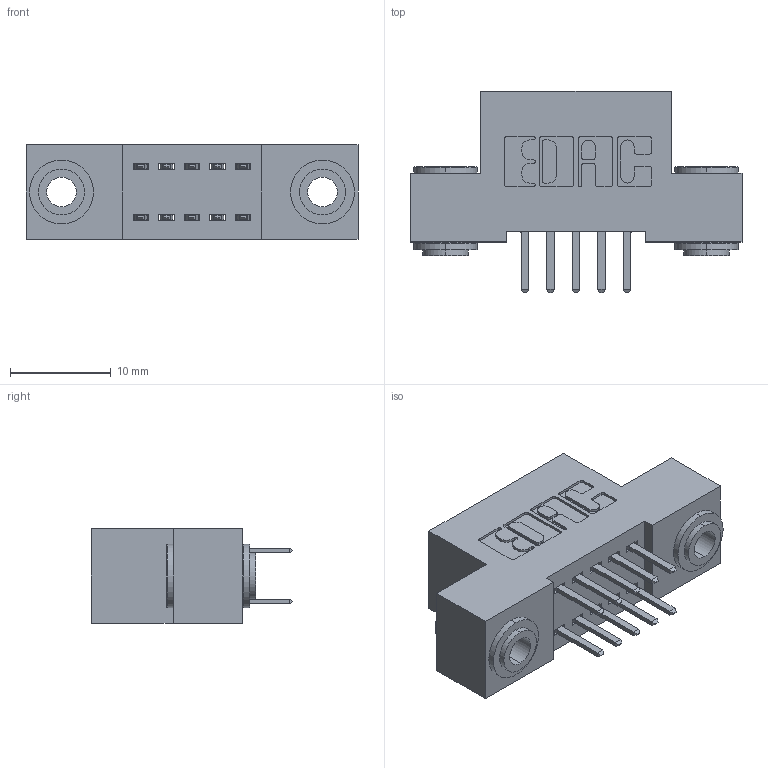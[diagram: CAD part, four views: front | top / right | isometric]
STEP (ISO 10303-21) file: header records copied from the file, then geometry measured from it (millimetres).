
FILE_DESCRIPTION (( 'STEP AP203' ), '1' );
FILE_NAME ('392-010-520-203.STEP', '2019-10-05T00:31:54', ( '' ), ( '' ), 'SwSTEP 2.0', 'SolidWorks 2016', '' );
FILE_SCHEMA (( 'CONFIG_CONTROL_DESIGN' ));
Length unit declared in the file: inch
Products named in the file (4): 342-250-002_345-250-002-102; 342 Part_.156 TH; 345-292-001_345-293-120; 392-010-520-203
Assembly tree (13 placements, depth 2):
  392-010-520-203
    342 Part_.156 TH
    345-292-001_345-293-120  x10
    342-250-002_345-250-002-102  x2
Bounding box: 33.02 x 20.02 x 9.4 mm (x, y, z)
Volume: 2810.1 mm3; surface area: 3866.2 mm2
Topology: 13 solids, 13 shells, 708 faces, 2005 edges, 1306 vertices
Faces by surface type: plane 456, cylinder 244, cone 8
Entity records: 8634 total; most frequent: CARTESIAN_POINT 1461, ORIENTED_EDGE 1378, DIRECTION 1335, EDGE_CURVE 689, LINE 533, VECTOR 533, VERTEX_POINT 454, AXIS2_PLACEMENT_3D 401
